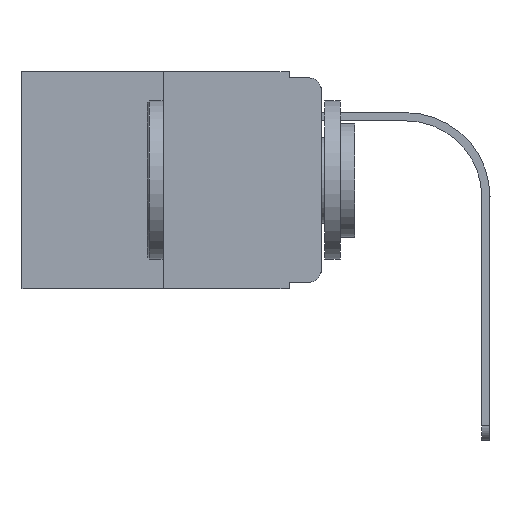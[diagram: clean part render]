
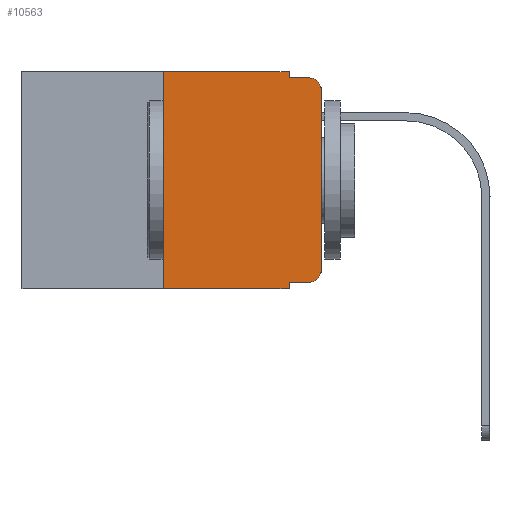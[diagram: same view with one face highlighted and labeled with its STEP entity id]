
A CAD part, left-side view. The second image highlights one B-rep face of the part: STEP entity #10563.
In plain terms, the highlighted planar face has unit normal (-1, 0, 0).
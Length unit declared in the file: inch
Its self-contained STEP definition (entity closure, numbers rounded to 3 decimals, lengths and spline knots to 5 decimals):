
#161 = CARTESIAN_POINT ( 'NONE',  ( 0., 0.051, 0. ) ) ;
#800 = ORIENTED_EDGE ( 'NONE', *, *, #12473, .F. ) ;
#966 = DIRECTION ( 'NONE',  ( 0., -1., 0. ) ) ;
#1173 = CARTESIAN_POINT ( 'NONE',  ( 0., 0.25, 0. ) ) ;
#1735 = CARTESIAN_POINT ( 'NONE',  ( 0., 0., 0. ) ) ;
#1806 = CARTESIAN_POINT ( 'NONE',  ( 0., 0.25, 0. ) ) ;
#1863 = DIRECTION ( 'NONE',  ( 0., -1., 0. ) ) ;
#1920 = VECTOR ( 'NONE', #19889, 39.37008 ) ;
#1992 = VERTEX_POINT ( 'NONE', #13991 ) ;
#2730 = CARTESIAN_POINT ( 'NONE',  ( 0., 0.051, -0.333 ) ) ;
#3010 = ORIENTED_EDGE ( 'NONE', *, *, #3954, .T. ) ;
#3295 = AXIS2_PLACEMENT_3D ( 'NONE', #14170, #14459, #6548 ) ;
#3954 = EDGE_CURVE ( 'NONE', #1992, #9696, #6758, .T. ) ;
#4227 = EDGE_CURVE ( 'NONE', #12486, #5633, #7487, .T. ) ;
#4265 = ORIENTED_EDGE ( 'NONE', *, *, #12707, .F. ) ;
#4708 = CARTESIAN_POINT ( 'NONE',  ( 0., 0.473, 0. ) ) ;
#4801 = CARTESIAN_POINT ( 'NONE',  ( 0., 0.051, -0.333 ) ) ;
#4805 = EDGE_CURVE ( 'NONE', #13287, #11528, #9682, .T. ) ;
#5056 = CARTESIAN_POINT ( 'NONE',  ( 0., 0.051, -0.01 ) ) ;
#5155 = CARTESIAN_POINT ( 'NONE',  ( 0., 0.02, -0.333 ) ) ;
#5336 = DIRECTION ( 'NONE',  ( 1., 0., 0. ) ) ;
#5495 = CARTESIAN_POINT ( 'NONE',  ( 0., 0.473, -0.343 ) ) ;
#5633 = VERTEX_POINT ( 'NONE', #16385 ) ;
#5888 = ORIENTED_EDGE ( 'NONE', *, *, #4227, .F. ) ;
#6306 = LINE ( 'NONE', #20059, #18987 ) ;
#6548 = DIRECTION ( 'NONE',  ( 0., 0., -1. ) ) ;
#6758 = LINE ( 'NONE', #1735, #18753 ) ;
#6965 = VECTOR ( 'NONE', #1863, 39.37008 ) ;
#7137 = AXIS2_PLACEMENT_3D ( 'NONE', #13279, #19515, #9871 ) ;
#7198 = ORIENTED_EDGE ( 'NONE', *, *, #12573, .T. ) ;
#7487 = LINE ( 'NONE', #4708, #1920 ) ;
#8125 = CIRCLE ( 'NONE', #7137, 0.02 ) ;
#8413 = ORIENTED_EDGE ( 'NONE', *, *, #13570, .T. ) ;
#8725 = CARTESIAN_POINT ( 'NONE',  ( 0., 0.051, -0.01 ) ) ;
#8756 = VERTEX_POINT ( 'NONE', #5155 ) ;
#8899 = DIRECTION ( 'NONE',  ( 0., -1., 0. ) ) ;
#9404 = ORIENTED_EDGE ( 'NONE', *, *, #10755, .T. ) ;
#9536 = EDGE_LOOP ( 'NONE', ( #3010, #9404, #10891, #800, #5888, #4265, #7198, #11634, #11543, #8413 ) ) ;
#9559 = CARTESIAN_POINT ( 'NONE',  ( 0., 0.051, -0.343 ) ) ;
#9607 = VECTOR ( 'NONE', #15257, 39.37008 ) ;
#9608 = VECTOR ( 'NONE', #9811, 39.37008 ) ;
#9682 = LINE ( 'NONE', #5056, #6965 ) ;
#9696 = VERTEX_POINT ( 'NONE', #10030 ) ;
#9811 = DIRECTION ( 'NONE',  ( 0., 0., -1. ) ) ;
#9871 = DIRECTION ( 'NONE',  ( 0., 0., -1. ) ) ;
#9940 = DIRECTION ( 'NONE',  ( 0., 0., 1. ) ) ;
#10030 = CARTESIAN_POINT ( 'NONE',  ( 0., 0., -0.03 ) ) ;
#10320 = LINE ( 'NONE', #5495, #10599 ) ;
#10563 = ADVANCED_FACE ( 'NONE', ( #14683 ), #13147, .F. ) ;
#10599 = VECTOR ( 'NONE', #966, 39.37008 ) ;
#10755 = EDGE_CURVE ( 'NONE', #9696, #11528, #17717, .T. ) ;
#10891 = ORIENTED_EDGE ( 'NONE', *, *, #4805, .F. ) ;
#11528 = VERTEX_POINT ( 'NONE', #16989 ) ;
#11543 = ORIENTED_EDGE ( 'NONE', *, *, #15853, .T. ) ;
#11597 = DIRECTION ( 'NONE',  ( 0., 0., -1. ) ) ;
#11634 = ORIENTED_EDGE ( 'NONE', *, *, #20259, .F. ) ;
#12164 = AXIS2_PLACEMENT_3D ( 'NONE', #19394, #5336, #11597 ) ;
#12407 = VERTEX_POINT ( 'NONE', #4801 ) ;
#12473 = EDGE_CURVE ( 'NONE', #5633, #13287, #15892, .T. ) ;
#12486 = VERTEX_POINT ( 'NONE', #1806 ) ;
#12573 = EDGE_CURVE ( 'NONE', #17612, #15245, #10320, .T. ) ;
#12707 = EDGE_CURVE ( 'NONE', #17612, #12486, #20165, .T. ) ;
#13147 = PLANE ( 'NONE',  #12164 ) ;
#13279 = CARTESIAN_POINT ( 'NONE',  ( 0., 0.02, -0.313 ) ) ;
#13287 = VERTEX_POINT ( 'NONE', #8725 ) ;
#13570 = EDGE_CURVE ( 'NONE', #8756, #1992, #8125, .T. ) ;
#13991 = CARTESIAN_POINT ( 'NONE',  ( 0., 0., -0.313 ) ) ;
#14170 = CARTESIAN_POINT ( 'NONE',  ( 0., 0.02, -0.03 ) ) ;
#14459 = DIRECTION ( 'NONE',  ( -1., 0., 0. ) ) ;
#14683 = FACE_OUTER_BOUND ( 'NONE', #9536, .T. ) ;
#14937 = CARTESIAN_POINT ( 'NONE',  ( 0., 0.25, -0.343 ) ) ;
#15245 = VERTEX_POINT ( 'NONE', #9559 ) ;
#15257 = DIRECTION ( 'NONE',  ( 0., 0., 1. ) ) ;
#15269 = LINE ( 'NONE', #2730, #19408 ) ;
#15853 = EDGE_CURVE ( 'NONE', #12407, #8756, #15269, .T. ) ;
#15892 = LINE ( 'NONE', #161, #9608 ) ;
#16385 = CARTESIAN_POINT ( 'NONE',  ( 0., 0.051, 0. ) ) ;
#16989 = CARTESIAN_POINT ( 'NONE',  ( 0., 0.02, -0.01 ) ) ;
#17298 = DIRECTION ( 'NONE',  ( 0., 0., -1. ) ) ;
#17612 = VERTEX_POINT ( 'NONE', #14937 ) ;
#17717 = CIRCLE ( 'NONE', #3295, 0.02 ) ;
#18753 = VECTOR ( 'NONE', #9940, 39.37008 ) ;
#18987 = VECTOR ( 'NONE', #17298, 39.37008 ) ;
#19394 = CARTESIAN_POINT ( 'NONE',  ( 0., 0.473, 0. ) ) ;
#19408 = VECTOR ( 'NONE', #8899, 39.37008 ) ;
#19515 = DIRECTION ( 'NONE',  ( -1., 0., 0. ) ) ;
#19889 = DIRECTION ( 'NONE',  ( 0., -1., 0. ) ) ;
#20059 = CARTESIAN_POINT ( 'NONE',  ( 0., 0.051, 0. ) ) ;
#20165 = LINE ( 'NONE', #1173, #9607 ) ;
#20259 = EDGE_CURVE ( 'NONE', #12407, #15245, #6306, .T. ) ;
